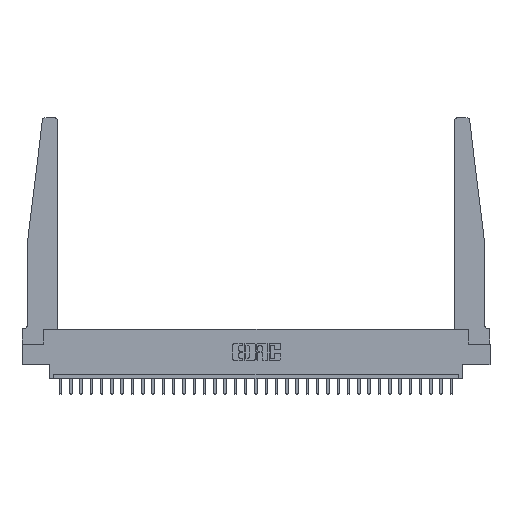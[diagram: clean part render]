
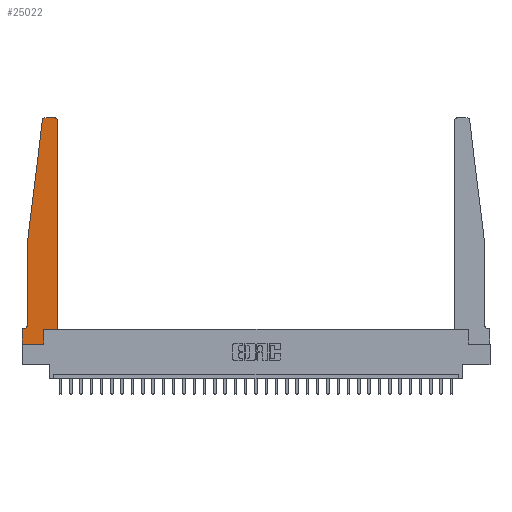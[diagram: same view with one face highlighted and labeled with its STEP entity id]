
A CAD part, top view. The second image highlights one B-rep face of the part: STEP entity #25022.
In plain terms, the highlighted planar face has unit normal (0, 0, 1).
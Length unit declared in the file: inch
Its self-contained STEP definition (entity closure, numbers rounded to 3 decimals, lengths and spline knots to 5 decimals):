
#60 = CARTESIAN_POINT ( 'NONE',  ( 0.2605, 0.18, 0.37 ) ) ;
#922 = VERTEX_POINT ( 'NONE', #6847 ) ;
#1089 = DIRECTION ( 'NONE',  ( 1., 0., 0. ) ) ;
#1181 = DIRECTION ( 'NONE',  ( -1., 0., 0. ) ) ;
#1412 = VERTEX_POINT ( 'NONE', #4516 ) ;
#1937 = VERTEX_POINT ( 'NONE', #24821 ) ;
#2151 = VECTOR ( 'NONE', #4819, 39.37008 ) ;
#2283 = VERTEX_POINT ( 'NONE', #27398 ) ;
#2477 = VECTOR ( 'NONE', #23598, 39.37008 ) ;
#2732 = DIRECTION ( 'NONE',  ( 1., 0., 0. ) ) ;
#2844 = LINE ( 'NONE', #12461, #2477 ) ;
#3347 = FACE_OUTER_BOUND ( 'NONE', #11775, .T. ) ;
#3440 = DIRECTION ( 'NONE',  ( -0.122, -0.992, 0. ) ) ;
#3820 = VECTOR ( 'NONE', #29518, 39.37008 ) ;
#4015 = EDGE_CURVE ( 'NONE', #1412, #922, #11135, .T. ) ;
#4516 = CARTESIAN_POINT ( 'NONE',  ( 0.27653, 2.75, 0.37 ) ) ;
#4586 = EDGE_CURVE ( 'NONE', #9006, #10855, #2844, .T. ) ;
#4608 = DIRECTION ( 'NONE',  ( 0., 0., 1. ) ) ;
#4655 = ORIENTED_EDGE ( 'NONE', *, *, #5610, .T. ) ;
#4819 = DIRECTION ( 'NONE',  ( 0., 1., 0. ) ) ;
#5610 = EDGE_CURVE ( 'NONE', #12753, #25421, #28157, .T. ) ;
#5689 = ORIENTED_EDGE ( 'NONE', *, *, #25849, .T. ) ;
#5810 = CIRCLE ( 'NONE', #11603, 0.05 ) ;
#6152 = ORIENTED_EDGE ( 'NONE', *, *, #17080, .T. ) ;
#6395 = EDGE_CURVE ( 'NONE', #24066, #2283, #9822, .T. ) ;
#6847 = CARTESIAN_POINT ( 'NONE',  ( 0.24675, 2.72367, 0.37 ) ) ;
#7144 = ORIENTED_EDGE ( 'NONE', *, *, #16262, .T. ) ;
#7228 = DIRECTION ( 'NONE',  ( 0., -1., 0. ) ) ;
#7273 = CARTESIAN_POINT ( 'NONE',  ( 0.395, 2.72, 0.37 ) ) ;
#7464 = DIRECTION ( 'NONE',  ( 0., 0., 1. ) ) ;
#7657 = DIRECTION ( 'NONE',  ( 1., 0., 0. ) ) ;
#7677 = LINE ( 'NONE', #15176, #11207 ) ;
#7740 = PLANE ( 'NONE',  #14087 ) ;
#7921 = CARTESIAN_POINT ( 'NONE',  ( 0.25, 2.75, 0.37 ) ) ;
#9006 = VERTEX_POINT ( 'NONE', #17380 ) ;
#9389 = CARTESIAN_POINT ( 'NONE',  ( 0.065, 0.2375, 0.37 ) ) ;
#9446 = ORIENTED_EDGE ( 'NONE', *, *, #29324, .T. ) ;
#9822 = LINE ( 'NONE', #27065, #3820 ) ;
#10014 = CARTESIAN_POINT ( 'NONE',  ( 0., 0.1875, 0.37 ) ) ;
#10076 = ORIENTED_EDGE ( 'NONE', *, *, #4586, .T. ) ;
#10855 = VERTEX_POINT ( 'NONE', #27699 ) ;
#11012 = LINE ( 'NONE', #23259, #2151 ) ;
#11135 = CIRCLE ( 'NONE', #27928, 0.03 ) ;
#11207 = VECTOR ( 'NONE', #24411, 39.37008 ) ;
#11422 = CARTESIAN_POINT ( 'NONE',  ( 0.2605, 0.18, 0.37 ) ) ;
#11603 = AXIS2_PLACEMENT_3D ( 'NONE', #20373, #27301, #24862 ) ;
#11672 = LINE ( 'NONE', #11422, #23157 ) ;
#11775 = EDGE_LOOP ( 'NONE', ( #6152, #14035, #7144, #4655, #29483, #9446, #10076, #5689, #15545, #26550, #14021, #17408 ) ) ;
#12461 = CARTESIAN_POINT ( 'NONE',  ( 0., 0., 0.37 ) ) ;
#12753 = VERTEX_POINT ( 'NONE', #27978 ) ;
#12796 = VECTOR ( 'NONE', #1181, 39.37008 ) ;
#13393 = VECTOR ( 'NONE', #7228, 39.37008 ) ;
#13885 = DIRECTION ( 'NONE',  ( 1., 0., 0. ) ) ;
#14021 = ORIENTED_EDGE ( 'NONE', *, *, #26908, .T. ) ;
#14035 = ORIENTED_EDGE ( 'NONE', *, *, #4015, .T. ) ;
#14087 = AXIS2_PLACEMENT_3D ( 'NONE', #10014, #14574, #1089 ) ;
#14574 = DIRECTION ( 'NONE',  ( 0., 0., 1. ) ) ;
#14707 = CARTESIAN_POINT ( 'NONE',  ( 0.065, 1.25, 0.37 ) ) ;
#15176 = CARTESIAN_POINT ( 'NONE',  ( 0.065, 0.1875, 0.37 ) ) ;
#15528 = CARTESIAN_POINT ( 'NONE',  ( 0.015, 0.1875, 0.37 ) ) ;
#15545 = ORIENTED_EDGE ( 'NONE', *, *, #19963, .T. ) ;
#16086 = DIRECTION ( 'NONE',  ( 0., 1., 0. ) ) ;
#16262 = EDGE_CURVE ( 'NONE', #922, #12753, #25299, .T. ) ;
#16295 = CARTESIAN_POINT ( 'NONE',  ( 0., 0., 0.37 ) ) ;
#16703 = CIRCLE ( 'NONE', #20122, 0.03 ) ;
#16721 = CARTESIAN_POINT ( 'NONE',  ( 0.425, 2.72, 0.37 ) ) ;
#17080 = EDGE_CURVE ( 'NONE', #1937, #1412, #25303, .T. ) ;
#17187 = EDGE_CURVE ( 'NONE', #20306, #1937, #16703, .T. ) ;
#17380 = CARTESIAN_POINT ( 'NONE',  ( 0., 0.1875, 0.37 ) ) ;
#17408 = ORIENTED_EDGE ( 'NONE', *, *, #17187, .T. ) ;
#17504 = VERTEX_POINT ( 'NONE', #15528 ) ;
#19229 = VECTOR ( 'NONE', #3440, 39.37008 ) ;
#19963 = EDGE_CURVE ( 'NONE', #26704, #24066, #11672, .T. ) ;
#20122 = AXIS2_PLACEMENT_3D ( 'NONE', #7273, #4608, #13885 ) ;
#20306 = VERTEX_POINT ( 'NONE', #16721 ) ;
#20373 = CARTESIAN_POINT ( 'NONE',  ( 0.015, 0.2375, 0.37 ) ) ;
#23100 = CARTESIAN_POINT ( 'NONE',  ( 0.065, 1.25, 0.37 ) ) ;
#23157 = VECTOR ( 'NONE', #16086, 39.37008 ) ;
#23259 = CARTESIAN_POINT ( 'NONE',  ( 0.425, 0.18, 0.37 ) ) ;
#23540 = CARTESIAN_POINT ( 'NONE',  ( 0.27653, 2.72, 0.37 ) ) ;
#23598 = DIRECTION ( 'NONE',  ( 0., -1., 0. ) ) ;
#24066 = VERTEX_POINT ( 'NONE', #60 ) ;
#24411 = DIRECTION ( 'NONE',  ( -1., 0., 0. ) ) ;
#24446 = CARTESIAN_POINT ( 'NONE',  ( 0.2605, 0., 0.37 ) ) ;
#24821 = CARTESIAN_POINT ( 'NONE',  ( 0.395, 2.75, 0.37 ) ) ;
#24862 = DIRECTION ( 'NONE',  ( -1., 0., 0. ) ) ;
#25022 = ADVANCED_FACE ( 'NONE', ( #3347 ), #7740, .T. ) ;
#25033 = EDGE_CURVE ( 'NONE', #25421, #17504, #5810, .T. ) ;
#25299 = LINE ( 'NONE', #14707, #19229 ) ;
#25303 = LINE ( 'NONE', #7921, #12796 ) ;
#25421 = VERTEX_POINT ( 'NONE', #9389 ) ;
#25849 = EDGE_CURVE ( 'NONE', #10855, #26704, #27539, .T. ) ;
#26550 = ORIENTED_EDGE ( 'NONE', *, *, #6395, .T. ) ;
#26704 = VERTEX_POINT ( 'NONE', #24446 ) ;
#26908 = EDGE_CURVE ( 'NONE', #2283, #20306, #11012, .T. ) ;
#27065 = CARTESIAN_POINT ( 'NONE',  ( 0.425, 0.18, 0.37 ) ) ;
#27185 = VECTOR ( 'NONE', #2732, 39.37008 ) ;
#27301 = DIRECTION ( 'NONE',  ( 0., 0., -1. ) ) ;
#27398 = CARTESIAN_POINT ( 'NONE',  ( 0.425, 0.18, 0.37 ) ) ;
#27539 = LINE ( 'NONE', #16295, #27185 ) ;
#27699 = CARTESIAN_POINT ( 'NONE',  ( 0., 0., 0.37 ) ) ;
#27928 = AXIS2_PLACEMENT_3D ( 'NONE', #23540, #7464, #7657 ) ;
#27978 = CARTESIAN_POINT ( 'NONE',  ( 0.065, 1.25, 0.37 ) ) ;
#28157 = LINE ( 'NONE', #23100, #13393 ) ;
#29324 = EDGE_CURVE ( 'NONE', #17504, #9006, #7677, .T. ) ;
#29483 = ORIENTED_EDGE ( 'NONE', *, *, #25033, .T. ) ;
#29518 = DIRECTION ( 'NONE',  ( 1., 0., 0. ) ) ;
